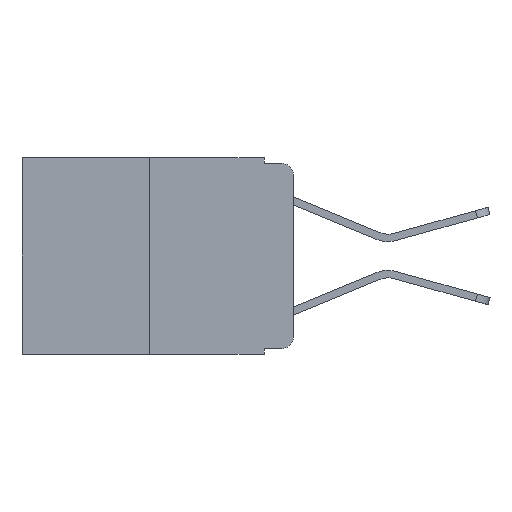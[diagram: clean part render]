
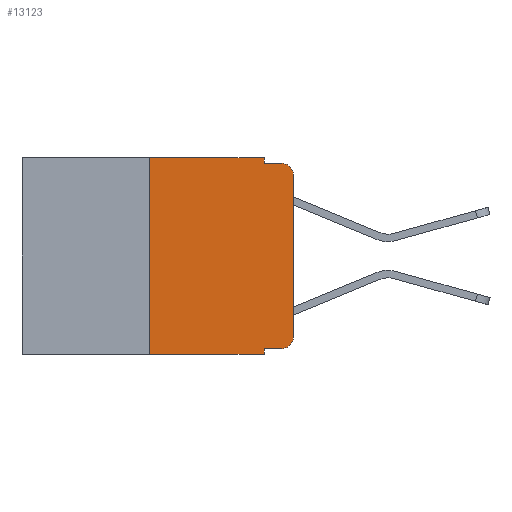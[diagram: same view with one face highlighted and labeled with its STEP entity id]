
A CAD part, left-side view. The second image highlights one B-rep face of the part: STEP entity #13123.
In plain terms, the highlighted planar face has unit normal (-1, 0, 0).
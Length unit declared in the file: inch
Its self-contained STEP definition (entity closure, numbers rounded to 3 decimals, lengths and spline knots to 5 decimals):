
#48 = CARTESIAN_POINT ( 'NONE',  ( 0., 0.473, 0. ) ) ;
#138 = EDGE_CURVE ( 'NONE', #4345, #9793, #7414, .T. ) ;
#212 = FACE_OUTER_BOUND ( 'NONE', #5940, .T. ) ;
#365 = DIRECTION ( 'NONE',  ( 0., 0., -1. ) ) ;
#501 = CARTESIAN_POINT ( 'NONE',  ( 0., 0.02, -0.03 ) ) ;
#934 = DIRECTION ( 'NONE',  ( 0., 0., 1. ) ) ;
#958 = ORIENTED_EDGE ( 'NONE', *, *, #1725, .F. ) ;
#1104 = LINE ( 'NONE', #48, #11730 ) ;
#1119 = DIRECTION ( 'NONE',  ( 0., -1., 0. ) ) ;
#1126 = VERTEX_POINT ( 'NONE', #3260 ) ;
#1162 = AXIS2_PLACEMENT_3D ( 'NONE', #8158, #9174, #13164 ) ;
#1554 = DIRECTION ( 'NONE',  ( -1., 0., 0. ) ) ;
#1564 = ORIENTED_EDGE ( 'NONE', *, *, #9511, .T. ) ;
#1674 = CARTESIAN_POINT ( 'NONE',  ( 0., 0.051, 0. ) ) ;
#1707 = CARTESIAN_POINT ( 'NONE',  ( 0., 0.051, 0. ) ) ;
#1725 = EDGE_CURVE ( 'NONE', #9793, #4428, #1104, .T. ) ;
#1869 = EDGE_CURVE ( 'NONE', #2634, #4860, #8657, .T. ) ;
#2041 = ORIENTED_EDGE ( 'NONE', *, *, #1869, .T. ) ;
#2051 = ORIENTED_EDGE ( 'NONE', *, *, #7408, .T. ) ;
#2565 = EDGE_CURVE ( 'NONE', #4428, #12354, #2846, .T. ) ;
#2634 = VERTEX_POINT ( 'NONE', #8139 ) ;
#2737 = ORIENTED_EDGE ( 'NONE', *, *, #11758, .T. ) ;
#2846 = LINE ( 'NONE', #1707, #7515 ) ;
#2859 = AXIS2_PLACEMENT_3D ( 'NONE', #501, #1554, #365 ) ;
#2961 = CARTESIAN_POINT ( 'NONE',  ( 0., 0.25, 0. ) ) ;
#3260 = CARTESIAN_POINT ( 'NONE',  ( 0., 0., -0.313 ) ) ;
#4123 = VERTEX_POINT ( 'NONE', #8137 ) ;
#4264 = EDGE_CURVE ( 'NONE', #12354, #4860, #6202, .T. ) ;
#4345 = VERTEX_POINT ( 'NONE', #6392 ) ;
#4428 = VERTEX_POINT ( 'NONE', #6054 ) ;
#4470 = CARTESIAN_POINT ( 'NONE',  ( 0., 0.051, -0.01 ) ) ;
#4572 = LINE ( 'NONE', #1674, #11182 ) ;
#4583 = LINE ( 'NONE', #9677, #7495 ) ;
#4667 = CARTESIAN_POINT ( 'NONE',  ( 0., 0.051, -0.333 ) ) ;
#4810 = DIRECTION ( 'NONE',  ( 0., 0., -1. ) ) ;
#4860 = VERTEX_POINT ( 'NONE', #10479 ) ;
#5331 = VERTEX_POINT ( 'NONE', #8185 ) ;
#5715 = VECTOR ( 'NONE', #11113, 39.37008 ) ;
#5940 = EDGE_LOOP ( 'NONE', ( #1564, #2041, #13131, #13128, #958, #12220, #10653, #9099, #2737, #2051 ) ) ;
#6054 = CARTESIAN_POINT ( 'NONE',  ( 0., 0.051, 0. ) ) ;
#6157 = LINE ( 'NONE', #4667, #7273 ) ;
#6202 = LINE ( 'NONE', #8355, #13113 ) ;
#6392 = CARTESIAN_POINT ( 'NONE',  ( 0., 0.25, -0.343 ) ) ;
#6695 = LINE ( 'NONE', #9031, #5715 ) ;
#6775 = DIRECTION ( 'NONE',  ( 0., -1., 0. ) ) ;
#7172 = CARTESIAN_POINT ( 'NONE',  ( 0., 0.25, 0. ) ) ;
#7250 = VECTOR ( 'NONE', #934, 39.37008 ) ;
#7273 = VECTOR ( 'NONE', #6775, 39.37008 ) ;
#7408 = EDGE_CURVE ( 'NONE', #11434, #1126, #10243, .T. ) ;
#7414 = LINE ( 'NONE', #2961, #7250 ) ;
#7495 = VECTOR ( 'NONE', #12834, 39.37008 ) ;
#7515 = VECTOR ( 'NONE', #9108, 39.37008 ) ;
#8137 = CARTESIAN_POINT ( 'NONE',  ( 0., 0.051, -0.343 ) ) ;
#8139 = CARTESIAN_POINT ( 'NONE',  ( 0., 0., -0.03 ) ) ;
#8158 = CARTESIAN_POINT ( 'NONE',  ( 0., 0.473, 0. ) ) ;
#8185 = CARTESIAN_POINT ( 'NONE',  ( 0., 0.051, -0.333 ) ) ;
#8355 = CARTESIAN_POINT ( 'NONE',  ( 0., 0.051, -0.01 ) ) ;
#8381 = CARTESIAN_POINT ( 'NONE',  ( 0., 0.02, -0.313 ) ) ;
#8397 = DIRECTION ( 'NONE',  ( 0., -1., 0. ) ) ;
#8657 = CIRCLE ( 'NONE', #2859, 0.02 ) ;
#9031 = CARTESIAN_POINT ( 'NONE',  ( 0., 0.473, -0.343 ) ) ;
#9099 = ORIENTED_EDGE ( 'NONE', *, *, #9568, .F. ) ;
#9108 = DIRECTION ( 'NONE',  ( 0., 0., -1. ) ) ;
#9174 = DIRECTION ( 'NONE',  ( 1., 0., 0. ) ) ;
#9511 = EDGE_CURVE ( 'NONE', #1126, #2634, #4583, .T. ) ;
#9568 = EDGE_CURVE ( 'NONE', #5331, #4123, #4572, .T. ) ;
#9634 = EDGE_CURVE ( 'NONE', #4345, #4123, #6695, .T. ) ;
#9677 = CARTESIAN_POINT ( 'NONE',  ( 0., 0., 0. ) ) ;
#9793 = VERTEX_POINT ( 'NONE', #7172 ) ;
#10158 = PLANE ( 'NONE',  #1162 ) ;
#10243 = CIRCLE ( 'NONE', #11713, 0.02 ) ;
#10248 = CARTESIAN_POINT ( 'NONE',  ( 0., 0.02, -0.333 ) ) ;
#10427 = DIRECTION ( 'NONE',  ( -1., 0., 0. ) ) ;
#10479 = CARTESIAN_POINT ( 'NONE',  ( 0., 0.02, -0.01 ) ) ;
#10653 = ORIENTED_EDGE ( 'NONE', *, *, #9634, .T. ) ;
#11113 = DIRECTION ( 'NONE',  ( 0., -1., 0. ) ) ;
#11182 = VECTOR ( 'NONE', #4810, 39.37008 ) ;
#11434 = VERTEX_POINT ( 'NONE', #10248 ) ;
#11713 = AXIS2_PLACEMENT_3D ( 'NONE', #8381, #10427, #12513 ) ;
#11730 = VECTOR ( 'NONE', #1119, 39.37008 ) ;
#11758 = EDGE_CURVE ( 'NONE', #5331, #11434, #6157, .T. ) ;
#12220 = ORIENTED_EDGE ( 'NONE', *, *, #138, .F. ) ;
#12354 = VERTEX_POINT ( 'NONE', #4470 ) ;
#12513 = DIRECTION ( 'NONE',  ( 0., 0., -1. ) ) ;
#12834 = DIRECTION ( 'NONE',  ( 0., 0., 1. ) ) ;
#13113 = VECTOR ( 'NONE', #8397, 39.37008 ) ;
#13123 = ADVANCED_FACE ( 'NONE', ( #212 ), #10158, .F. ) ;
#13128 = ORIENTED_EDGE ( 'NONE', *, *, #2565, .F. ) ;
#13131 = ORIENTED_EDGE ( 'NONE', *, *, #4264, .F. ) ;
#13164 = DIRECTION ( 'NONE',  ( 0., 0., -1. ) ) ;
